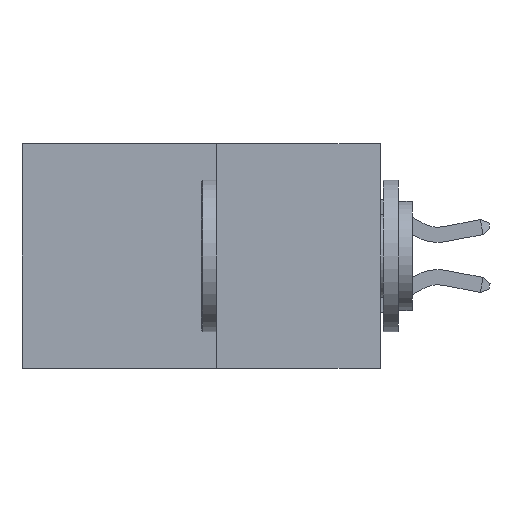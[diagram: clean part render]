
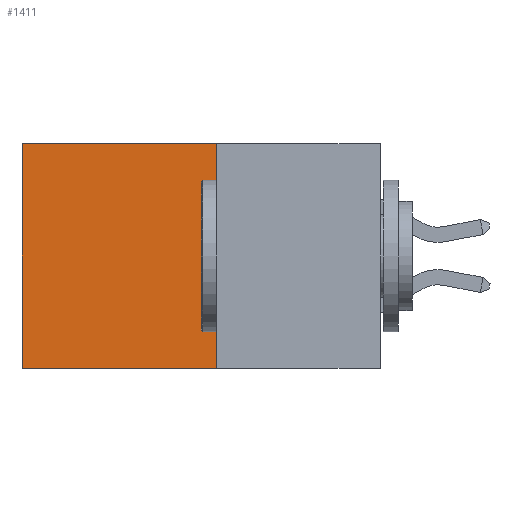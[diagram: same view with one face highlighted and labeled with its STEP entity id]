
A CAD part, left-side view. The second image highlights one B-rep face of the part: STEP entity #1411.
In plain terms, the highlighted planar face has unit normal (-1, 0, 0).
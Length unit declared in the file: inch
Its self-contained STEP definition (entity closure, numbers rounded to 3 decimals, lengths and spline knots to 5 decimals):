
#521 = PLANE ( 'NONE',  #8004 ) ;
#1056 = EDGE_LOOP ( 'NONE', ( #2163, #8266, #8527, #2622 ) ) ;
#1411 = ADVANCED_FACE ( 'NONE', ( #4218 ), #521, .F. ) ;
#1574 = LINE ( 'NONE', #4586, #5285 ) ;
#1969 = DIRECTION ( 'NONE',  ( 0., 0., -1. ) ) ;
#2030 = VERTEX_POINT ( 'NONE', #9653 ) ;
#2123 = EDGE_CURVE ( 'NONE', #4241, #2030, #4779, .T. ) ;
#2163 = ORIENTED_EDGE ( 'NONE', *, *, #4281, .T. ) ;
#2185 = CARTESIAN_POINT ( 'NONE',  ( 0.277, 0.27, -0.37 ) ) ;
#2424 = DIRECTION ( 'NONE',  ( 0., 0., -1. ) ) ;
#2465 = CARTESIAN_POINT ( 'NONE',  ( 0.277, 0.59, -0.37 ) ) ;
#2580 = CARTESIAN_POINT ( 'NONE',  ( 0.277, 0.27, -0.37 ) ) ;
#2622 = ORIENTED_EDGE ( 'NONE', *, *, #9313, .T. ) ;
#3057 = CARTESIAN_POINT ( 'NONE',  ( 0.277, 0.27, -0.37 ) ) ;
#3662 = VECTOR ( 'NONE', #4045, 39.37008 ) ;
#3840 = DIRECTION ( 'NONE',  ( 0., 1., 0. ) ) ;
#3929 = CARTESIAN_POINT ( 'NONE',  ( 0.277, 0.27, 0. ) ) ;
#4045 = DIRECTION ( 'NONE',  ( 0., 1., 0. ) ) ;
#4218 = FACE_OUTER_BOUND ( 'NONE', #1056, .T. ) ;
#4241 = VERTEX_POINT ( 'NONE', #3929 ) ;
#4281 = EDGE_CURVE ( 'NONE', #7009, #8869, #7684, .T. ) ;
#4586 = CARTESIAN_POINT ( 'NONE',  ( 0.277, 0.27, 0. ) ) ;
#4779 = LINE ( 'NONE', #3057, #6580 ) ;
#4890 = CARTESIAN_POINT ( 'NONE',  ( 0.277, 0.59, 0. ) ) ;
#5285 = VECTOR ( 'NONE', #3840, 39.37008 ) ;
#6580 = VECTOR ( 'NONE', #1969, 39.37008 ) ;
#7009 = VERTEX_POINT ( 'NONE', #4890 ) ;
#7059 = DIRECTION ( 'NONE',  ( 1., 0., 0. ) ) ;
#7133 = DIRECTION ( 'NONE',  ( 0., 0., -1. ) ) ;
#7673 = EDGE_CURVE ( 'NONE', #2030, #8869, #8001, .T. ) ;
#7684 = LINE ( 'NONE', #2465, #9543 ) ;
#8001 = LINE ( 'NONE', #2580, #3662 ) ;
#8004 = AXIS2_PLACEMENT_3D ( 'NONE', #2185, #7059, #7133 ) ;
#8266 = ORIENTED_EDGE ( 'NONE', *, *, #7673, .F. ) ;
#8527 = ORIENTED_EDGE ( 'NONE', *, *, #2123, .F. ) ;
#8803 = CARTESIAN_POINT ( 'NONE',  ( 0.277, 0.59, -0.37 ) ) ;
#8869 = VERTEX_POINT ( 'NONE', #8803 ) ;
#9313 = EDGE_CURVE ( 'NONE', #4241, #7009, #1574, .T. ) ;
#9543 = VECTOR ( 'NONE', #2424, 39.37008 ) ;
#9653 = CARTESIAN_POINT ( 'NONE',  ( 0.277, 0.27, -0.37 ) ) ;
